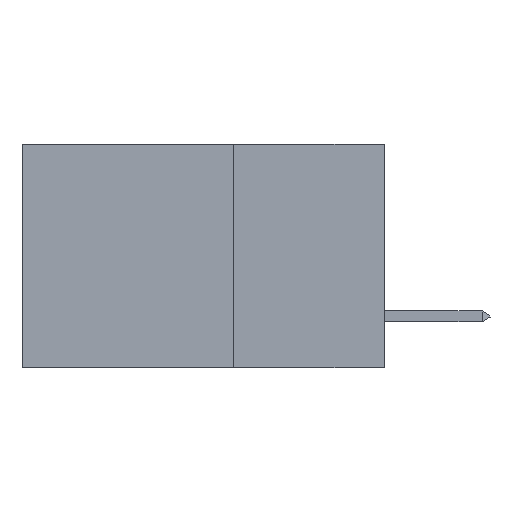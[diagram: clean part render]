
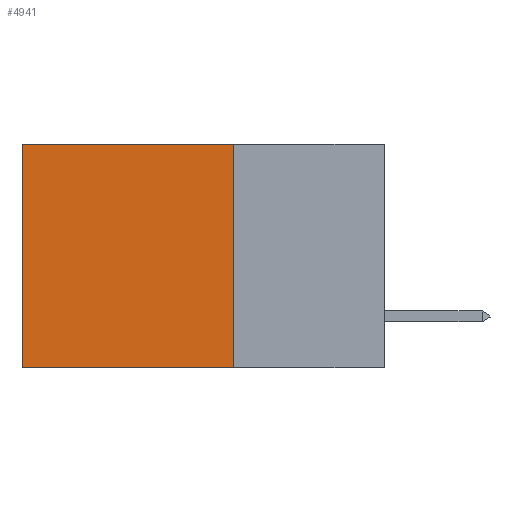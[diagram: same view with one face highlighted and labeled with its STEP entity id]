
A CAD part, left-side view. The second image highlights one B-rep face of the part: STEP entity #4941.
In plain terms, the highlighted planar face has unit normal (-1, 0, 0).
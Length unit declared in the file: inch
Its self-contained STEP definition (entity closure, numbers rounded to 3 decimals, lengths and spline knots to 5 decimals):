
#143 = CARTESIAN_POINT ( 'NONE',  ( 0.2875, 0.6, 0. ) ) ;
#190 = DIRECTION ( 'NONE',  ( 0., 1., 0. ) ) ;
#408 = CARTESIAN_POINT ( 'NONE',  ( 0.2875, 0.25, -0.37 ) ) ;
#491 = VECTOR ( 'NONE', #190, 39.37008 ) ;
#701 = FACE_OUTER_BOUND ( 'NONE', #2083, .T. ) ;
#1376 = LINE ( 'NONE', #10331, #491 ) ;
#1593 = DIRECTION ( 'NONE',  ( 0., 0., -1. ) ) ;
#1852 = ORIENTED_EDGE ( 'NONE', *, *, #7114, .T. ) ;
#1890 = DIRECTION ( 'NONE',  ( 0., 0., -1. ) ) ;
#2083 = EDGE_LOOP ( 'NONE', ( #8312, #8536, #10106, #1852 ) ) ;
#2452 = VERTEX_POINT ( 'NONE', #3326 ) ;
#2600 = CARTESIAN_POINT ( 'NONE',  ( 0.2875, 0.25, 0. ) ) ;
#3313 = DIRECTION ( 'NONE',  ( 1., 0., 0. ) ) ;
#3326 = CARTESIAN_POINT ( 'NONE',  ( 0.2875, 0.6, -0.37 ) ) ;
#3389 = VECTOR ( 'NONE', #1593, 39.37008 ) ;
#3391 = DIRECTION ( 'NONE',  ( 0., 0., -1. ) ) ;
#3533 = VERTEX_POINT ( 'NONE', #11473 ) ;
#4932 = AXIS2_PLACEMENT_3D ( 'NONE', #5153, #3313, #3391 ) ;
#4941 = ADVANCED_FACE ( 'NONE', ( #701 ), #8823, .F. ) ;
#5153 = CARTESIAN_POINT ( 'NONE',  ( 0.2875, 0.25, 0. ) ) ;
#6976 = VECTOR ( 'NONE', #1890, 39.37008 ) ;
#7114 = EDGE_CURVE ( 'NONE', #10259, #10071, #1376, .T. ) ;
#7357 = EDGE_CURVE ( 'NONE', #10071, #2452, #8278, .T. ) ;
#8028 = VECTOR ( 'NONE', #10590, 39.37008 ) ;
#8083 = EDGE_CURVE ( 'NONE', #10259, #3533, #8970, .T. ) ;
#8278 = LINE ( 'NONE', #8926, #3389 ) ;
#8312 = ORIENTED_EDGE ( 'NONE', *, *, #7357, .T. ) ;
#8536 = ORIENTED_EDGE ( 'NONE', *, *, #11602, .F. ) ;
#8823 = PLANE ( 'NONE',  #4932 ) ;
#8926 = CARTESIAN_POINT ( 'NONE',  ( 0.2875, 0.6, 0. ) ) ;
#8970 = LINE ( 'NONE', #11290, #6976 ) ;
#10071 = VERTEX_POINT ( 'NONE', #143 ) ;
#10106 = ORIENTED_EDGE ( 'NONE', *, *, #8083, .F. ) ;
#10259 = VERTEX_POINT ( 'NONE', #2600 ) ;
#10331 = CARTESIAN_POINT ( 'NONE',  ( 0.2875, 0.25, 0. ) ) ;
#10506 = LINE ( 'NONE', #408, #8028 ) ;
#10590 = DIRECTION ( 'NONE',  ( 0., 1., 0. ) ) ;
#11290 = CARTESIAN_POINT ( 'NONE',  ( 0.2875, 0.25, 0. ) ) ;
#11473 = CARTESIAN_POINT ( 'NONE',  ( 0.2875, 0.25, -0.37 ) ) ;
#11602 = EDGE_CURVE ( 'NONE', #3533, #2452, #10506, .T. ) ;
